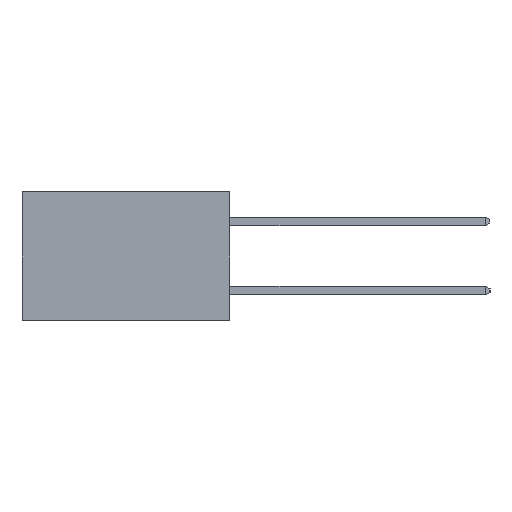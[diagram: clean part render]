
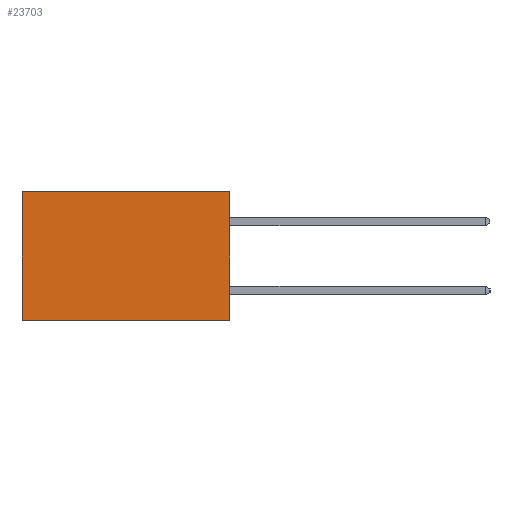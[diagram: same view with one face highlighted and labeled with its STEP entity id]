
A CAD part, left-side view. The second image highlights one B-rep face of the part: STEP entity #23703.
In plain terms, the highlighted planar face has unit normal (-1, 0, 0).
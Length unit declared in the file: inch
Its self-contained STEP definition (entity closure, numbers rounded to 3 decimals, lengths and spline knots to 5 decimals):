
#472 = LINE ( 'NONE', #14048, #10938 ) ;
#895 = DIRECTION ( 'NONE',  ( 1., 0., 0. ) ) ;
#2405 = CARTESIAN_POINT ( 'NONE',  ( 0.2615, 0., -0.37 ) ) ;
#3730 = VERTEX_POINT ( 'NONE', #5037 ) ;
#4352 = LINE ( 'NONE', #5175, #18556 ) ;
#5037 = CARTESIAN_POINT ( 'NONE',  ( 0.2615, 0.6, -0.37 ) ) ;
#5096 = LINE ( 'NONE', #17641, #14824 ) ;
#5175 = CARTESIAN_POINT ( 'NONE',  ( 0.2615, 0., -0.37 ) ) ;
#5816 = CARTESIAN_POINT ( 'NONE',  ( 0.2615, 0., -0.37 ) ) ;
#5849 = FACE_OUTER_BOUND ( 'NONE', #22399, .T. ) ;
#6318 = EDGE_CURVE ( 'NONE', #18417, #8086, #5096, .T. ) ;
#6469 = LINE ( 'NONE', #2405, #15568 ) ;
#7123 = ORIENTED_EDGE ( 'NONE', *, *, #7465, .F. ) ;
#7144 = DIRECTION ( 'NONE',  ( 0., 0., -1. ) ) ;
#7241 = AXIS2_PLACEMENT_3D ( 'NONE', #12633, #895, #14588 ) ;
#7465 = EDGE_CURVE ( 'NONE', #18417, #9183, #4352, .T. ) ;
#8031 = EDGE_CURVE ( 'NONE', #9183, #3730, #6469, .T. ) ;
#8086 = VERTEX_POINT ( 'NONE', #10467 ) ;
#9183 = VERTEX_POINT ( 'NONE', #5816 ) ;
#9592 = ORIENTED_EDGE ( 'NONE', *, *, #14436, .T. ) ;
#10467 = CARTESIAN_POINT ( 'NONE',  ( 0.2615, 0.6, 0. ) ) ;
#10938 = VECTOR ( 'NONE', #15988, 39.37008 ) ;
#12300 = DIRECTION ( 'NONE',  ( 0., 1., 0. ) ) ;
#12633 = CARTESIAN_POINT ( 'NONE',  ( 0.2615, 0., -0.37 ) ) ;
#12989 = ORIENTED_EDGE ( 'NONE', *, *, #8031, .F. ) ;
#14048 = CARTESIAN_POINT ( 'NONE',  ( 0.2615, 0.6, -0.37 ) ) ;
#14436 = EDGE_CURVE ( 'NONE', #8086, #3730, #472, .T. ) ;
#14588 = DIRECTION ( 'NONE',  ( 0., 0., -1. ) ) ;
#14824 = VECTOR ( 'NONE', #21488, 39.37008 ) ;
#15568 = VECTOR ( 'NONE', #12300, 39.37008 ) ;
#15988 = DIRECTION ( 'NONE',  ( 0., 0., -1. ) ) ;
#17442 = CARTESIAN_POINT ( 'NONE',  ( 0.2615, 0., 0. ) ) ;
#17641 = CARTESIAN_POINT ( 'NONE',  ( 0.2615, 0., 0. ) ) ;
#18417 = VERTEX_POINT ( 'NONE', #17442 ) ;
#18556 = VECTOR ( 'NONE', #7144, 39.37008 ) ;
#21488 = DIRECTION ( 'NONE',  ( 0., 1., 0. ) ) ;
#22167 = PLANE ( 'NONE',  #7241 ) ;
#22399 = EDGE_LOOP ( 'NONE', ( #9592, #12989, #7123, #24093 ) ) ;
#23703 = ADVANCED_FACE ( 'NONE', ( #5849 ), #22167, .F. ) ;
#24093 = ORIENTED_EDGE ( 'NONE', *, *, #6318, .T. ) ;
